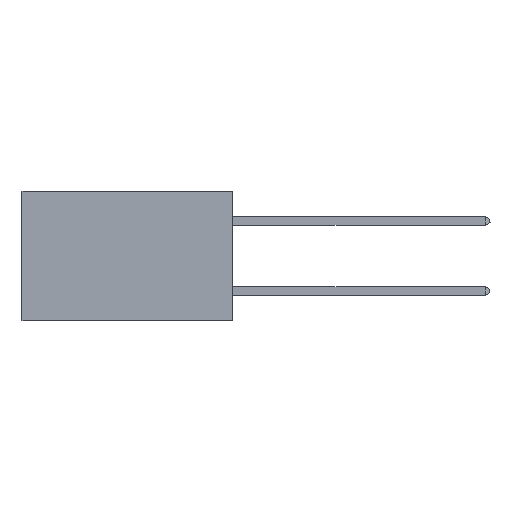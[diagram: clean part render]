
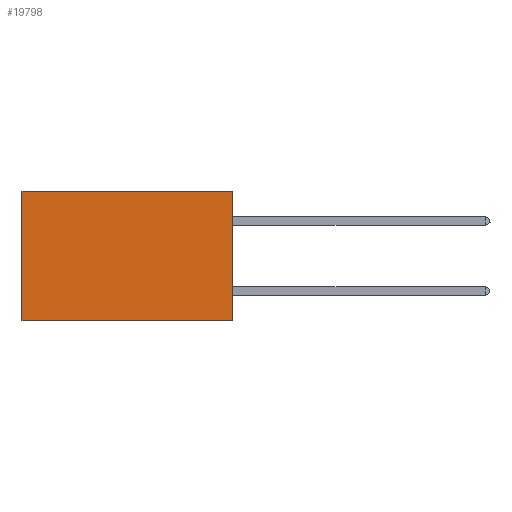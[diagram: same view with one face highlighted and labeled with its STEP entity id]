
A CAD part, left-side view. The second image highlights one B-rep face of the part: STEP entity #19798.
In plain terms, the highlighted planar face has unit normal (-1, 0, 0).
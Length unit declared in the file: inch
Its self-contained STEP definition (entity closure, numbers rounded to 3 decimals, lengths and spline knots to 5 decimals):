
#514 = EDGE_CURVE ( 'NONE', #11655, #9180, #12846, .T. ) ;
#1308 = CARTESIAN_POINT ( 'NONE',  ( 0.2875, 0., 0. ) ) ;
#1645 = DIRECTION ( 'NONE',  ( 0., 0., -1. ) ) ;
#2347 = ORIENTED_EDGE ( 'NONE', *, *, #15808, .F. ) ;
#3229 = VECTOR ( 'NONE', #10305, 39.37008 ) ;
#4439 = VECTOR ( 'NONE', #23028, 39.37008 ) ;
#5217 = CARTESIAN_POINT ( 'NONE',  ( 0.2875, 0.6, -0.37 ) ) ;
#7189 = CARTESIAN_POINT ( 'NONE',  ( 0.2875, 0., 0. ) ) ;
#7560 = DIRECTION ( 'NONE',  ( 1., 0., 0. ) ) ;
#8235 = AXIS2_PLACEMENT_3D ( 'NONE', #22082, #7560, #9626 ) ;
#8357 = VECTOR ( 'NONE', #1645, 39.37008 ) ;
#8545 = LINE ( 'NONE', #20389, #21337 ) ;
#9070 = CARTESIAN_POINT ( 'NONE',  ( 0.2875, 0.6, 0. ) ) ;
#9180 = VERTEX_POINT ( 'NONE', #22926 ) ;
#9626 = DIRECTION ( 'NONE',  ( 0., 0., -1. ) ) ;
#9993 = CARTESIAN_POINT ( 'NONE',  ( 0.2875, 0., -0.37 ) ) ;
#10305 = DIRECTION ( 'NONE',  ( 0., 1., 0. ) ) ;
#10544 = FACE_OUTER_BOUND ( 'NONE', #17484, .T. ) ;
#11655 = VERTEX_POINT ( 'NONE', #7189 ) ;
#12782 = PLANE ( 'NONE',  #8235 ) ;
#12846 = LINE ( 'NONE', #1308, #4439 ) ;
#13047 = ORIENTED_EDGE ( 'NONE', *, *, #14106, .T. ) ;
#14106 = EDGE_CURVE ( 'NONE', #9180, #14648, #21958, .T. ) ;
#14648 = VERTEX_POINT ( 'NONE', #5217 ) ;
#15637 = LINE ( 'NONE', #9993, #3229 ) ;
#15808 = EDGE_CURVE ( 'NONE', #18330, #14648, #15637, .T. ) ;
#17484 = EDGE_LOOP ( 'NONE', ( #13047, #2347, #21015, #22755 ) ) ;
#17657 = CARTESIAN_POINT ( 'NONE',  ( 0.2875, 0., -0.37 ) ) ;
#18330 = VERTEX_POINT ( 'NONE', #17657 ) ;
#19798 = ADVANCED_FACE ( 'NONE', ( #10544 ), #12782, .F. ) ;
#20350 = EDGE_CURVE ( 'NONE', #11655, #18330, #8545, .T. ) ;
#20389 = CARTESIAN_POINT ( 'NONE',  ( 0.2875, 0., 0. ) ) ;
#20465 = DIRECTION ( 'NONE',  ( 0., 0., -1. ) ) ;
#21015 = ORIENTED_EDGE ( 'NONE', *, *, #20350, .F. ) ;
#21337 = VECTOR ( 'NONE', #20465, 39.37008 ) ;
#21958 = LINE ( 'NONE', #9070, #8357 ) ;
#22082 = CARTESIAN_POINT ( 'NONE',  ( 0.2875, 0., 0. ) ) ;
#22755 = ORIENTED_EDGE ( 'NONE', *, *, #514, .T. ) ;
#22926 = CARTESIAN_POINT ( 'NONE',  ( 0.2875, 0.6, 0. ) ) ;
#23028 = DIRECTION ( 'NONE',  ( 0., 1., 0. ) ) ;
